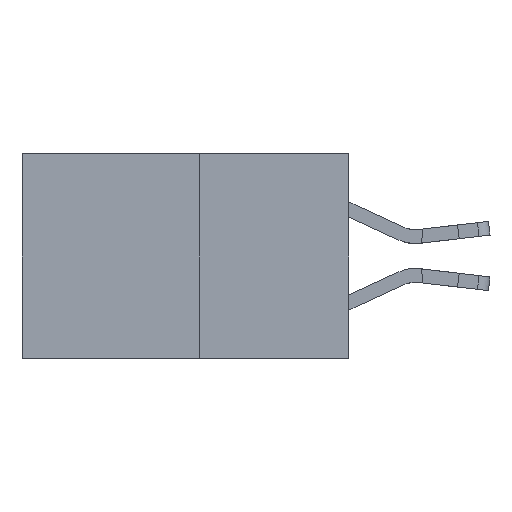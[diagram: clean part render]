
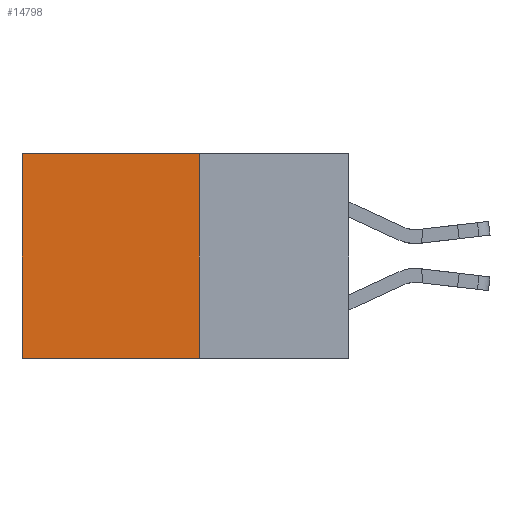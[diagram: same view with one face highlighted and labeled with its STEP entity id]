
A CAD part, left-side view. The second image highlights one B-rep face of the part: STEP entity #14798.
In plain terms, the highlighted planar face has unit normal (-1, 0, 0).
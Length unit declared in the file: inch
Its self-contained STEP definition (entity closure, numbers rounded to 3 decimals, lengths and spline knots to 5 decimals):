
#46 = DIRECTION ( 'NONE',  ( 1., 0., 0. ) ) ;
#718 = CARTESIAN_POINT ( 'NONE',  ( 0.277, 0.27, -0.37 ) ) ;
#3003 = EDGE_CURVE ( 'NONE', #28563, #29083, #18596, .T. ) ;
#4500 = EDGE_LOOP ( 'NONE', ( #12450, #10612, #7240, #12475 ) ) ;
#5522 = DIRECTION ( 'NONE',  ( 0., 0., -1. ) ) ;
#6913 = VECTOR ( 'NONE', #5522, 39.37008 ) ;
#7240 = ORIENTED_EDGE ( 'NONE', *, *, #8068, .F. ) ;
#7592 = DIRECTION ( 'NONE',  ( 0., 0., -1. ) ) ;
#7599 = EDGE_CURVE ( 'NONE', #19358, #18975, #27939, .T. ) ;
#8068 = EDGE_CURVE ( 'NONE', #19358, #28563, #19546, .T. ) ;
#10612 = ORIENTED_EDGE ( 'NONE', *, *, #3003, .F. ) ;
#10846 = CARTESIAN_POINT ( 'NONE',  ( 0.277, 0.59, -0.37 ) ) ;
#12450 = ORIENTED_EDGE ( 'NONE', *, *, #29438, .T. ) ;
#12475 = ORIENTED_EDGE ( 'NONE', *, *, #7599, .T. ) ;
#12852 = CARTESIAN_POINT ( 'NONE',  ( 0.277, 0.27, -0.37 ) ) ;
#14330 = CARTESIAN_POINT ( 'NONE',  ( 0.277, 0.27, -0.37 ) ) ;
#14364 = CARTESIAN_POINT ( 'NONE',  ( 0.277, 0.27, -0.37 ) ) ;
#14798 = ADVANCED_FACE ( 'NONE', ( #23484 ), #16014, .F. ) ;
#16014 = PLANE ( 'NONE',  #17001 ) ;
#16727 = DIRECTION ( 'NONE',  ( 0., 0., -1. ) ) ;
#17001 = AXIS2_PLACEMENT_3D ( 'NONE', #14330, #46, #16727 ) ;
#18596 = LINE ( 'NONE', #14364, #25501 ) ;
#18975 = VERTEX_POINT ( 'NONE', #20813 ) ;
#19205 = DIRECTION ( 'NONE',  ( 0., 1., 0. ) ) ;
#19358 = VERTEX_POINT ( 'NONE', #21162 ) ;
#19444 = CARTESIAN_POINT ( 'NONE',  ( 0.277, 0.59, -0.37 ) ) ;
#19546 = LINE ( 'NONE', #718, #6913 ) ;
#20813 = CARTESIAN_POINT ( 'NONE',  ( 0.277, 0.59, 0. ) ) ;
#21162 = CARTESIAN_POINT ( 'NONE',  ( 0.277, 0.27, 0. ) ) ;
#22524 = VECTOR ( 'NONE', #27373, 39.37008 ) ;
#23484 = FACE_OUTER_BOUND ( 'NONE', #4500, .T. ) ;
#25075 = CARTESIAN_POINT ( 'NONE',  ( 0.277, 0.27, 0. ) ) ;
#25501 = VECTOR ( 'NONE', #19205, 39.37008 ) ;
#27373 = DIRECTION ( 'NONE',  ( 0., 1., 0. ) ) ;
#27939 = LINE ( 'NONE', #25075, #22524 ) ;
#28563 = VERTEX_POINT ( 'NONE', #12852 ) ;
#28993 = VECTOR ( 'NONE', #7592, 39.37008 ) ;
#29083 = VERTEX_POINT ( 'NONE', #10846 ) ;
#29438 = EDGE_CURVE ( 'NONE', #18975, #29083, #29722, .T. ) ;
#29722 = LINE ( 'NONE', #19444, #28993 ) ;
